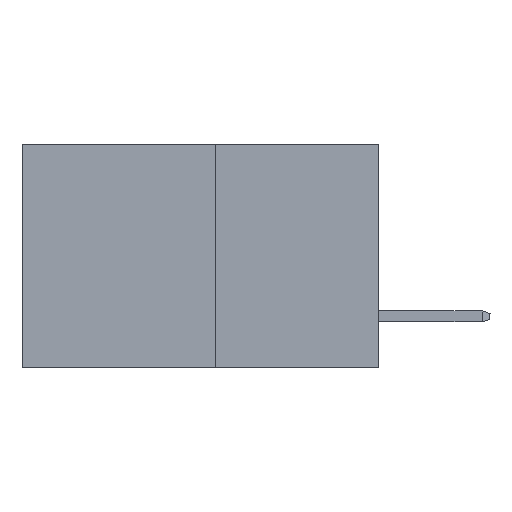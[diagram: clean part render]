
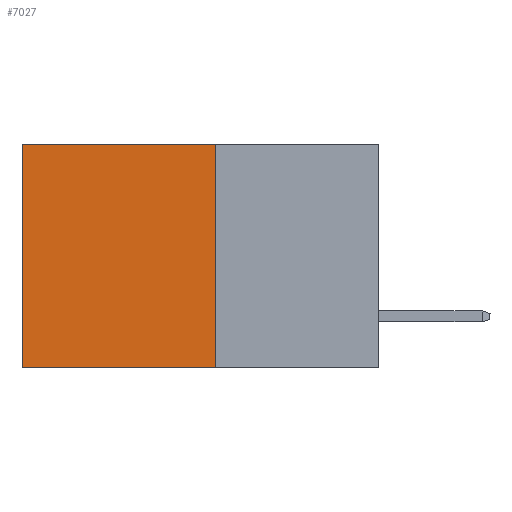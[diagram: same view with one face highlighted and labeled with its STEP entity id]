
A CAD part, left-side view. The second image highlights one B-rep face of the part: STEP entity #7027.
In plain terms, the highlighted planar face has unit normal (-1, 0, 0).
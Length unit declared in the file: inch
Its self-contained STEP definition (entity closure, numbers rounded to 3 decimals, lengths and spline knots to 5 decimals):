
#208 = EDGE_CURVE ( 'NONE', #6856, #2019, #4068, .T. ) ;
#287 = EDGE_CURVE ( 'NONE', #2019, #4812, #3150, .T. ) ;
#756 = CARTESIAN_POINT ( 'NONE',  ( 0.277, 0.27, -0.37 ) ) ;
#788 = LINE ( 'NONE', #756, #10144 ) ;
#863 = DIRECTION ( 'NONE',  ( 1., 0., 0. ) ) ;
#991 = ORIENTED_EDGE ( 'NONE', *, *, #287, .T. ) ;
#1459 = EDGE_CURVE ( 'NONE', #6856, #11389, #788, .T. ) ;
#1842 = VECTOR ( 'NONE', #5046, 39.37008 ) ;
#2019 = VERTEX_POINT ( 'NONE', #10571 ) ;
#3150 = LINE ( 'NONE', #3186, #10302 ) ;
#3186 = CARTESIAN_POINT ( 'NONE',  ( 0.277, 0.59, -0.37 ) ) ;
#3288 = CARTESIAN_POINT ( 'NONE',  ( 0.277, 0.27, 0. ) ) ;
#3492 = DIRECTION ( 'NONE',  ( 0., 0., -1. ) ) ;
#3657 = FACE_OUTER_BOUND ( 'NONE', #5157, .T. ) ;
#3788 = ORIENTED_EDGE ( 'NONE', *, *, #208, .T. ) ;
#4068 = LINE ( 'NONE', #7022, #1842 ) ;
#4812 = VERTEX_POINT ( 'NONE', #8905 ) ;
#5046 = DIRECTION ( 'NONE',  ( 0., 1., 0. ) ) ;
#5075 = DIRECTION ( 'NONE',  ( 0., 0., -1. ) ) ;
#5157 = EDGE_LOOP ( 'NONE', ( #991, #7240, #9633, #3788 ) ) ;
#6287 = LINE ( 'NONE', #7245, #8714 ) ;
#6596 = AXIS2_PLACEMENT_3D ( 'NONE', #7194, #863, #5075 ) ;
#6856 = VERTEX_POINT ( 'NONE', #3288 ) ;
#7022 = CARTESIAN_POINT ( 'NONE',  ( 0.277, 0.27, 0. ) ) ;
#7027 = ADVANCED_FACE ( 'NONE', ( #3657 ), #8294, .F. ) ;
#7194 = CARTESIAN_POINT ( 'NONE',  ( 0.277, 0.27, -0.37 ) ) ;
#7240 = ORIENTED_EDGE ( 'NONE', *, *, #9252, .F. ) ;
#7245 = CARTESIAN_POINT ( 'NONE',  ( 0.277, 0.27, -0.37 ) ) ;
#8147 = DIRECTION ( 'NONE',  ( 0., 1., 0. ) ) ;
#8294 = PLANE ( 'NONE',  #6596 ) ;
#8534 = DIRECTION ( 'NONE',  ( 0., 0., -1. ) ) ;
#8714 = VECTOR ( 'NONE', #8147, 39.37008 ) ;
#8905 = CARTESIAN_POINT ( 'NONE',  ( 0.277, 0.59, -0.37 ) ) ;
#8928 = CARTESIAN_POINT ( 'NONE',  ( 0.277, 0.27, -0.37 ) ) ;
#9252 = EDGE_CURVE ( 'NONE', #11389, #4812, #6287, .T. ) ;
#9633 = ORIENTED_EDGE ( 'NONE', *, *, #1459, .F. ) ;
#10144 = VECTOR ( 'NONE', #3492, 39.37008 ) ;
#10302 = VECTOR ( 'NONE', #8534, 39.37008 ) ;
#10571 = CARTESIAN_POINT ( 'NONE',  ( 0.277, 0.59, 0. ) ) ;
#11389 = VERTEX_POINT ( 'NONE', #8928 ) ;
